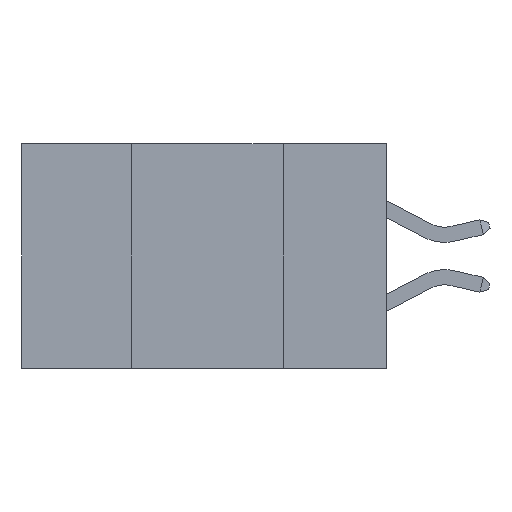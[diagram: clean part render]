
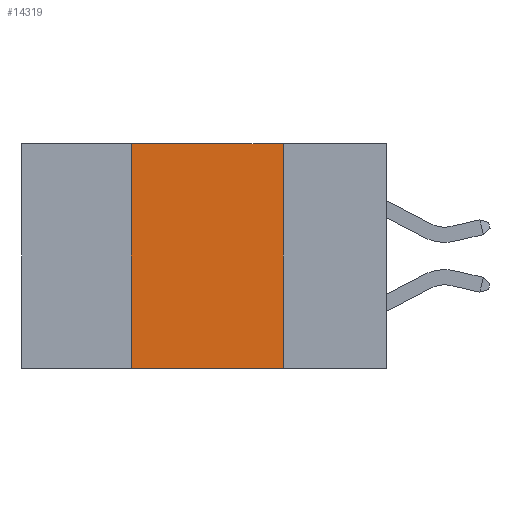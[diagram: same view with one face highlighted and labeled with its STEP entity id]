
A CAD part, left-side view. The second image highlights one B-rep face of the part: STEP entity #14319.
In plain terms, the highlighted planar face has unit normal (-1, 0, 0).
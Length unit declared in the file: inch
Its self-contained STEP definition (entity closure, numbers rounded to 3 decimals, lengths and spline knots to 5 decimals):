
#290 = VECTOR ( 'NONE', #15319, 39.37008 ) ;
#1388 = CARTESIAN_POINT ( 'NONE',  ( 0., 0.17, 0. ) ) ;
#1474 = AXIS2_PLACEMENT_3D ( 'NONE', #13348, #15042, #5079 ) ;
#1749 = PLANE ( 'NONE',  #1474 ) ;
#2025 = CARTESIAN_POINT ( 'NONE',  ( 0., 0.42, 0. ) ) ;
#2486 = EDGE_CURVE ( 'NONE', #8347, #14185, #6102, .T. ) ;
#3291 = CARTESIAN_POINT ( 'NONE',  ( 0., 0.17, -0.37 ) ) ;
#4693 = EDGE_CURVE ( 'NONE', #17633, #12995, #12668, .T. ) ;
#5079 = DIRECTION ( 'NONE',  ( 0., 0., -1. ) ) ;
#5305 = EDGE_LOOP ( 'NONE', ( #10376, #12605, #13836, #20227 ) ) ;
#5566 = VECTOR ( 'NONE', #5603, 39.37008 ) ;
#5603 = DIRECTION ( 'NONE',  ( 0., -1., 0. ) ) ;
#6102 = LINE ( 'NONE', #19858, #5566 ) ;
#6650 = CARTESIAN_POINT ( 'NONE',  ( 0., 0.42, 0. ) ) ;
#8347 = VERTEX_POINT ( 'NONE', #6650 ) ;
#10376 = ORIENTED_EDGE ( 'NONE', *, *, #13592, .F. ) ;
#10603 = FACE_OUTER_BOUND ( 'NONE', #5305, .T. ) ;
#11904 = LINE ( 'NONE', #17918, #19618 ) ;
#12143 = VECTOR ( 'NONE', #17653, 39.37008 ) ;
#12466 = EDGE_CURVE ( 'NONE', #17633, #8347, #13497, .T. ) ;
#12605 = ORIENTED_EDGE ( 'NONE', *, *, #2486, .F. ) ;
#12668 = LINE ( 'NONE', #14272, #12143 ) ;
#12995 = VERTEX_POINT ( 'NONE', #3291 ) ;
#13348 = CARTESIAN_POINT ( 'NONE',  ( 0., 0.6, 0. ) ) ;
#13497 = LINE ( 'NONE', #2025, #290 ) ;
#13592 = EDGE_CURVE ( 'NONE', #14185, #12995, #11904, .T. ) ;
#13836 = ORIENTED_EDGE ( 'NONE', *, *, #12466, .F. ) ;
#14185 = VERTEX_POINT ( 'NONE', #1388 ) ;
#14272 = CARTESIAN_POINT ( 'NONE',  ( 0., 0.6, -0.37 ) ) ;
#14319 = ADVANCED_FACE ( 'NONE', ( #10603 ), #1749, .F. ) ;
#15042 = DIRECTION ( 'NONE',  ( 1., 0., 0. ) ) ;
#15319 = DIRECTION ( 'NONE',  ( 0., 0., 1. ) ) ;
#17633 = VERTEX_POINT ( 'NONE', #21159 ) ;
#17653 = DIRECTION ( 'NONE',  ( 0., -1., 0. ) ) ;
#17918 = CARTESIAN_POINT ( 'NONE',  ( 0., 0.17, 0. ) ) ;
#19526 = DIRECTION ( 'NONE',  ( 0., 0., -1. ) ) ;
#19618 = VECTOR ( 'NONE', #19526, 39.37008 ) ;
#19858 = CARTESIAN_POINT ( 'NONE',  ( 0., 0.6, 0. ) ) ;
#20227 = ORIENTED_EDGE ( 'NONE', *, *, #4693, .T. ) ;
#21159 = CARTESIAN_POINT ( 'NONE',  ( 0., 0.42, -0.37 ) ) ;
